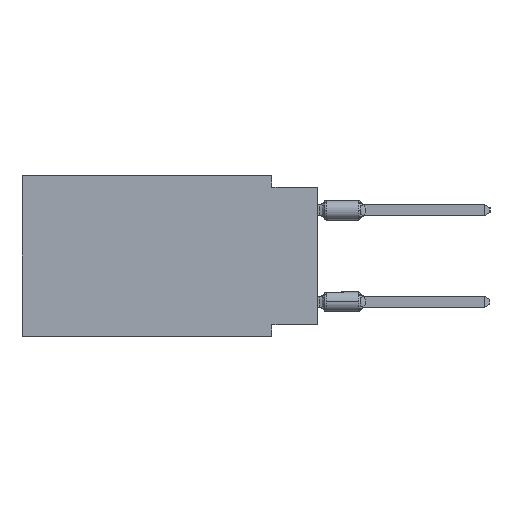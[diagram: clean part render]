
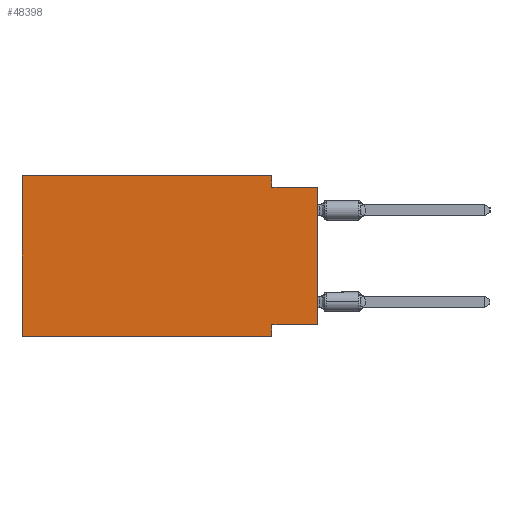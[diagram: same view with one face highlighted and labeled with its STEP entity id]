
A CAD part, left-side view. The second image highlights one B-rep face of the part: STEP entity #48398.
In plain terms, the highlighted planar face has unit normal (-1, 0, 0).
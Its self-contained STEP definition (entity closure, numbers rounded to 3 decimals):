
#1 = VECTOR ( 'NONE', #35983, 1000. ) ;
#583 = ORIENTED_EDGE ( 'NONE', *, *, #12567, .F. ) ;
#905 = EDGE_CURVE ( 'NONE', #7273, #33683, #59354, .T. ) ;
#1024 = DIRECTION ( 'NONE',  ( 1., 0., 0. ) ) ;
#2920 = LINE ( 'NONE', #22733, #60402 ) ;
#3281 = VECTOR ( 'NONE', #25886, 1000. ) ;
#4220 = LINE ( 'NONE', #24034, #1 ) ;
#5782 = ORIENTED_EDGE ( 'NONE', *, *, #59621, .T. ) ;
#5894 = PLANE ( 'NONE',  #27218 ) ;
#6641 = VERTEX_POINT ( 'NONE', #18608 ) ;
#6888 = CARTESIAN_POINT ( 'NONE',  ( 0., 0., -8.255 ) ) ;
#7273 = VERTEX_POINT ( 'NONE', #11052 ) ;
#9366 = EDGE_LOOP ( 'NONE', ( #18962, #37588, #36835, #47337, #23883, #5782, #28615, #583 ) ) ;
#10582 = CARTESIAN_POINT ( 'NONE',  ( 0., 0., -0.635 ) ) ;
#11052 = CARTESIAN_POINT ( 'NONE',  ( 0., 16.383, -8.89 ) ) ;
#11066 = VERTEX_POINT ( 'NONE', #56576 ) ;
#11138 = CARTESIAN_POINT ( 'NONE',  ( 0., 2.54, -0.635 ) ) ;
#12030 = CARTESIAN_POINT ( 'NONE',  ( 0., 16.383, 0. ) ) ;
#12567 = EDGE_CURVE ( 'NONE', #62724, #6641, #50372, .T. ) ;
#15189 = VECTOR ( 'NONE', #30262, 1000. ) ;
#15511 = CARTESIAN_POINT ( 'NONE',  ( 0., 2.54, -8.89 ) ) ;
#15557 = CARTESIAN_POINT ( 'NONE',  ( 0., 16.383, -8.89 ) ) ;
#15885 = LINE ( 'NONE', #15557, #50003 ) ;
#16198 = VERTEX_POINT ( 'NONE', #32806 ) ;
#16284 = FACE_OUTER_BOUND ( 'NONE', #9366, .T. ) ;
#18608 = CARTESIAN_POINT ( 'NONE',  ( 0., 2.54, -8.255 ) ) ;
#18962 = ORIENTED_EDGE ( 'NONE', *, *, #59380, .T. ) ;
#20738 = EDGE_CURVE ( 'NONE', #33683, #11066, #21448, .T. ) ;
#21448 = LINE ( 'NONE', #12030, #42977 ) ;
#22147 = DIRECTION ( 'NONE',  ( 0., -1., 0. ) ) ;
#22733 = CARTESIAN_POINT ( 'NONE',  ( 0., 0., 0. ) ) ;
#23883 = ORIENTED_EDGE ( 'NONE', *, *, #905, .F. ) ;
#24034 = CARTESIAN_POINT ( 'NONE',  ( 0., 2.54, 0. ) ) ;
#25701 = CARTESIAN_POINT ( 'NONE',  ( 0., 16.383, 0. ) ) ;
#25886 = DIRECTION ( 'NONE',  ( 0., 0., -1. ) ) ;
#26432 = CARTESIAN_POINT ( 'NONE',  ( 0., 0., -8.255 ) ) ;
#27218 = AXIS2_PLACEMENT_3D ( 'NONE', #25701, #1024, #55842 ) ;
#28418 = EDGE_CURVE ( 'NONE', #11066, #39823, #4220, .T. ) ;
#28615 = ORIENTED_EDGE ( 'NONE', *, *, #54954, .F. ) ;
#30262 = DIRECTION ( 'NONE',  ( 0., 1., 0. ) ) ;
#32806 = CARTESIAN_POINT ( 'NONE',  ( 0., 2.54, -8.89 ) ) ;
#33683 = VERTEX_POINT ( 'NONE', #39997 ) ;
#35983 = DIRECTION ( 'NONE',  ( 0., 0., -1. ) ) ;
#36025 = DIRECTION ( 'NONE',  ( 0., -1., 0. ) ) ;
#36835 = ORIENTED_EDGE ( 'NONE', *, *, #28418, .F. ) ;
#37588 = ORIENTED_EDGE ( 'NONE', *, *, #56016, .F. ) ;
#38614 = VERTEX_POINT ( 'NONE', #10582 ) ;
#39197 = CARTESIAN_POINT ( 'NONE',  ( 0., 16.383, 0. ) ) ;
#39750 = VECTOR ( 'NONE', #39857, 1000. ) ;
#39823 = VERTEX_POINT ( 'NONE', #11138 ) ;
#39857 = DIRECTION ( 'NONE',  ( 0., 0., 1. ) ) ;
#39997 = CARTESIAN_POINT ( 'NONE',  ( 0., 16.383, 0. ) ) ;
#42977 = VECTOR ( 'NONE', #36025, 1000. ) ;
#44061 = LINE ( 'NONE', #61725, #48950 ) ;
#44691 = LINE ( 'NONE', #15511, #3281 ) ;
#44735 = DIRECTION ( 'NONE',  ( 0., -1., 0. ) ) ;
#47337 = ORIENTED_EDGE ( 'NONE', *, *, #20738, .F. ) ;
#47684 = DIRECTION ( 'NONE',  ( 0., 0., 1. ) ) ;
#48398 = ADVANCED_FACE ( 'NONE', ( #16284 ), #5894, .F. ) ;
#48950 = VECTOR ( 'NONE', #22147, 1000. ) ;
#50003 = VECTOR ( 'NONE', #44735, 1000. ) ;
#50372 = LINE ( 'NONE', #6888, #15189 ) ;
#54954 = EDGE_CURVE ( 'NONE', #6641, #16198, #44691, .T. ) ;
#55842 = DIRECTION ( 'NONE',  ( 0., 0., -1. ) ) ;
#56016 = EDGE_CURVE ( 'NONE', #39823, #38614, #44061, .T. ) ;
#56576 = CARTESIAN_POINT ( 'NONE',  ( 0., 2.54, 0. ) ) ;
#59354 = LINE ( 'NONE', #39197, #39750 ) ;
#59380 = EDGE_CURVE ( 'NONE', #62724, #38614, #2920, .T. ) ;
#59621 = EDGE_CURVE ( 'NONE', #7273, #16198, #15885, .T. ) ;
#60402 = VECTOR ( 'NONE', #47684, 1000. ) ;
#61725 = CARTESIAN_POINT ( 'NONE',  ( 0., 0., -0.635 ) ) ;
#62724 = VERTEX_POINT ( 'NONE', #26432 ) ;
